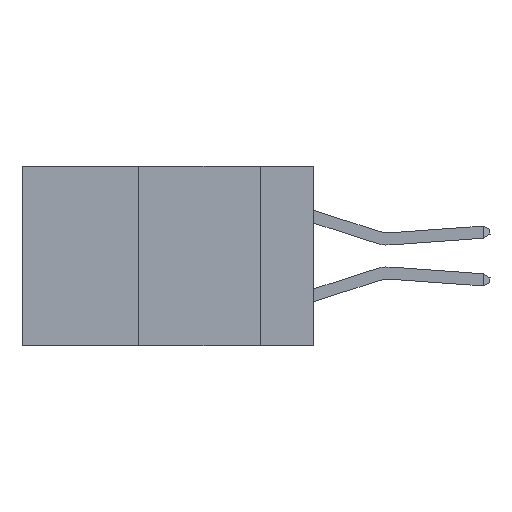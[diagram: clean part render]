
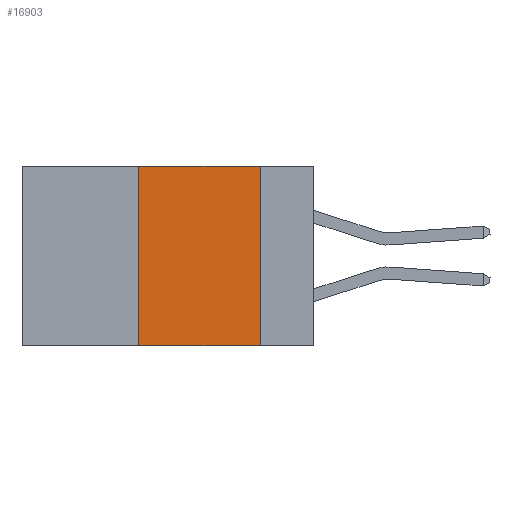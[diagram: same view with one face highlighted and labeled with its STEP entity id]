
A CAD part, left-side view. The second image highlights one B-rep face of the part: STEP entity #16903.
In plain terms, the highlighted planar face has unit normal (-1, 0, 0).
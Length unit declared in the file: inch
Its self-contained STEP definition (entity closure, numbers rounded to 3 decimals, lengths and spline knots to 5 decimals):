
#734 = LINE ( 'NONE', #5933, #20333 ) ;
#2073 = LINE ( 'NONE', #2383, #19703 ) ;
#2383 = CARTESIAN_POINT ( 'NONE',  ( 0., 0.6, 0. ) ) ;
#2726 = ORIENTED_EDGE ( 'NONE', *, *, #2879, .F. ) ;
#2879 = EDGE_CURVE ( 'NONE', #6425, #2932, #2073, .T. ) ;
#2932 = VERTEX_POINT ( 'NONE', #31744 ) ;
#3326 = LINE ( 'NONE', #12646, #3656 ) ;
#3656 = VECTOR ( 'NONE', #25140, 39.37008 ) ;
#4770 = DIRECTION ( 'NONE',  ( 0., -1., 0. ) ) ;
#5029 = ORIENTED_EDGE ( 'NONE', *, *, #18489, .F. ) ;
#5411 = ORIENTED_EDGE ( 'NONE', *, *, #16002, .T. ) ;
#5933 = CARTESIAN_POINT ( 'NONE',  ( 0., 0.36, 0. ) ) ;
#5981 = CARTESIAN_POINT ( 'NONE',  ( 0., 0.11, -0.37 ) ) ;
#6425 = VERTEX_POINT ( 'NONE', #27980 ) ;
#10546 = VERTEX_POINT ( 'NONE', #5981 ) ;
#11111 = LINE ( 'NONE', #30632, #14621 ) ;
#11890 = EDGE_LOOP ( 'NONE', ( #28045, #2726, #5029, #5411 ) ) ;
#12646 = CARTESIAN_POINT ( 'NONE',  ( 0., 0.6, -0.37 ) ) ;
#13567 = DIRECTION ( 'NONE',  ( 0., 0., 1. ) ) ;
#14621 = VECTOR ( 'NONE', #28421, 39.37008 ) ;
#16002 = EDGE_CURVE ( 'NONE', #31326, #10546, #3326, .T. ) ;
#16903 = ADVANCED_FACE ( 'NONE', ( #22892 ), #19061, .F. ) ;
#18489 = EDGE_CURVE ( 'NONE', #31326, #6425, #734, .T. ) ;
#19061 = PLANE ( 'NONE',  #20616 ) ;
#19703 = VECTOR ( 'NONE', #4770, 39.37008 ) ;
#20333 = VECTOR ( 'NONE', #13567, 39.37008 ) ;
#20616 = AXIS2_PLACEMENT_3D ( 'NONE', #29446, #26589, #21361 ) ;
#21361 = DIRECTION ( 'NONE',  ( 0., 0., -1. ) ) ;
#21630 = EDGE_CURVE ( 'NONE', #2932, #10546, #11111, .T. ) ;
#22892 = FACE_OUTER_BOUND ( 'NONE', #11890, .T. ) ;
#25140 = DIRECTION ( 'NONE',  ( 0., -1., 0. ) ) ;
#26589 = DIRECTION ( 'NONE',  ( 1., 0., 0. ) ) ;
#27980 = CARTESIAN_POINT ( 'NONE',  ( 0., 0.36, 0. ) ) ;
#28045 = ORIENTED_EDGE ( 'NONE', *, *, #21630, .F. ) ;
#28421 = DIRECTION ( 'NONE',  ( 0., 0., -1. ) ) ;
#29446 = CARTESIAN_POINT ( 'NONE',  ( 0., 0.6, 0. ) ) ;
#30558 = CARTESIAN_POINT ( 'NONE',  ( 0., 0.36, -0.37 ) ) ;
#30632 = CARTESIAN_POINT ( 'NONE',  ( 0., 0.11, 0. ) ) ;
#31326 = VERTEX_POINT ( 'NONE', #30558 ) ;
#31744 = CARTESIAN_POINT ( 'NONE',  ( 0., 0.11, 0. ) ) ;
